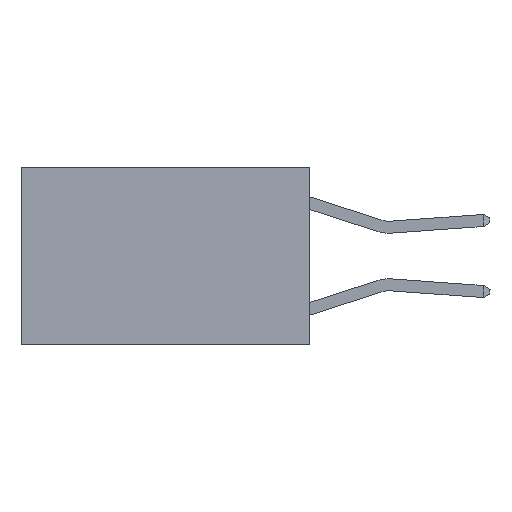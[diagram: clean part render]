
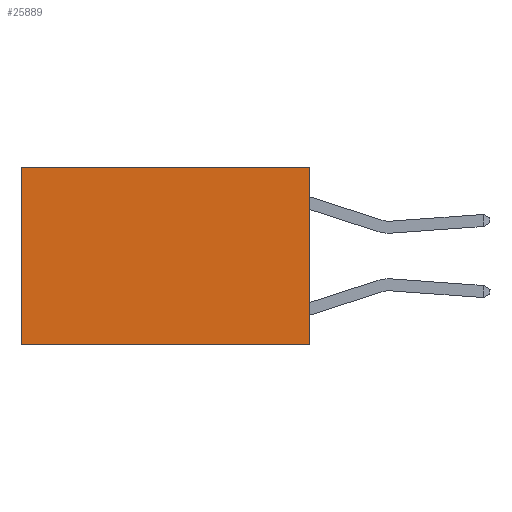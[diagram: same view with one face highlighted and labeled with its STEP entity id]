
A CAD part, left-side view. The second image highlights one B-rep face of the part: STEP entity #25889.
In plain terms, the highlighted planar face has unit normal (-1, 0, 0).
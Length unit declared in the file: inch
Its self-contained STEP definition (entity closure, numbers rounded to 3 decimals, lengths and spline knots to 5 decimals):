
#4 = DIRECTION ( 'NONE',  ( 0., 1., 0. ) ) ;
#292 = DIRECTION ( 'NONE',  ( 0., 0., -1. ) ) ;
#1619 = VECTOR ( 'NONE', #9804, 39.37008 ) ;
#3197 = CARTESIAN_POINT ( 'NONE',  ( 0.2625, 0.6, -0.37 ) ) ;
#3949 = VERTEX_POINT ( 'NONE', #7519 ) ;
#4975 = PLANE ( 'NONE',  #30066 ) ;
#5786 = LINE ( 'NONE', #30301, #29194 ) ;
#6204 = EDGE_CURVE ( 'NONE', #3949, #25675, #5786, .T. ) ;
#6884 = DIRECTION ( 'NONE',  ( 0., 0., -1. ) ) ;
#7078 = LINE ( 'NONE', #28107, #25040 ) ;
#7183 = FACE_OUTER_BOUND ( 'NONE', #17468, .T. ) ;
#7519 = CARTESIAN_POINT ( 'NONE',  ( 0.2625, 0., 0. ) ) ;
#7752 = ORIENTED_EDGE ( 'NONE', *, *, #11426, .T. ) ;
#8419 = CARTESIAN_POINT ( 'NONE',  ( 0.2625, 0., -0.37 ) ) ;
#8975 = CARTESIAN_POINT ( 'NONE',  ( 0.2625, 0.6, 0. ) ) ;
#9685 = ORIENTED_EDGE ( 'NONE', *, *, #26475, .F. ) ;
#9804 = DIRECTION ( 'NONE',  ( 0., 0., -1. ) ) ;
#10034 = VERTEX_POINT ( 'NONE', #3197 ) ;
#10713 = ORIENTED_EDGE ( 'NONE', *, *, #21321, .F. ) ;
#11426 = EDGE_CURVE ( 'NONE', #25675, #10034, #14119, .T. ) ;
#11609 = ORIENTED_EDGE ( 'NONE', *, *, #6204, .T. ) ;
#14119 = LINE ( 'NONE', #28508, #1619 ) ;
#14394 = DIRECTION ( 'NONE',  ( 1., 0., 0. ) ) ;
#17468 = EDGE_LOOP ( 'NONE', ( #7752, #10713, #9685, #11609 ) ) ;
#18692 = DIRECTION ( 'NONE',  ( 0., 1., 0. ) ) ;
#21321 = EDGE_CURVE ( 'NONE', #24209, #10034, #7078, .T. ) ;
#22169 = VECTOR ( 'NONE', #6884, 39.37008 ) ;
#24209 = VERTEX_POINT ( 'NONE', #8419 ) ;
#25040 = VECTOR ( 'NONE', #4, 39.37008 ) ;
#25517 = CARTESIAN_POINT ( 'NONE',  ( 0.2625, 0., 0. ) ) ;
#25675 = VERTEX_POINT ( 'NONE', #8975 ) ;
#25889 = ADVANCED_FACE ( 'NONE', ( #7183 ), #4975, .F. ) ;
#26475 = EDGE_CURVE ( 'NONE', #3949, #24209, #28361, .T. ) ;
#28107 = CARTESIAN_POINT ( 'NONE',  ( 0.2625, 0., -0.37 ) ) ;
#28361 = LINE ( 'NONE', #25517, #22169 ) ;
#28384 = CARTESIAN_POINT ( 'NONE',  ( 0.2625, 0., 0. ) ) ;
#28508 = CARTESIAN_POINT ( 'NONE',  ( 0.2625, 0.6, 0. ) ) ;
#29194 = VECTOR ( 'NONE', #18692, 39.37008 ) ;
#30066 = AXIS2_PLACEMENT_3D ( 'NONE', #28384, #14394, #292 ) ;
#30301 = CARTESIAN_POINT ( 'NONE',  ( 0.2625, 0., 0. ) ) ;
